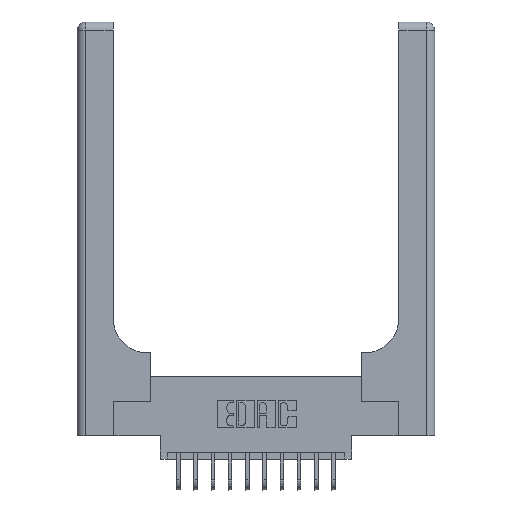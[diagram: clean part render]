
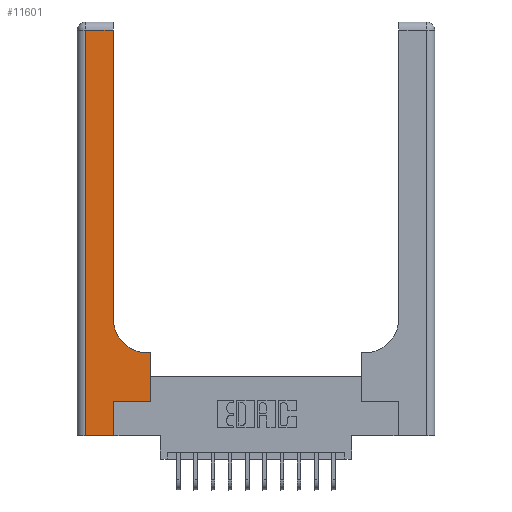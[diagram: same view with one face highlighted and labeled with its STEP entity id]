
A CAD part, top view. The second image highlights one B-rep face of the part: STEP entity #11601.
In plain terms, the highlighted planar face has unit normal (0, 0, 1).
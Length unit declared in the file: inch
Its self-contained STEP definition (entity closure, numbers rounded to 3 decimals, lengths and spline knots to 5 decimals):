
#465 = DIRECTION ( 'NONE',  ( 0., 1., 0. ) ) ;
#601 = PLANE ( 'NONE',  #8319 ) ;
#725 = ORIENTED_EDGE ( 'NONE', *, *, #13886, .T. ) ;
#1067 = EDGE_LOOP ( 'NONE', ( #1439, #725, #13092, #6729, #8405, #2641, #15620, #2859, #9228 ) ) ;
#1168 = VECTOR ( 'NONE', #14982, 39.37008 ) ;
#1403 = VERTEX_POINT ( 'NONE', #11383 ) ;
#1439 = ORIENTED_EDGE ( 'NONE', *, *, #6930, .T. ) ;
#1854 = LINE ( 'NONE', #16345, #11852 ) ;
#1896 = CIRCLE ( 'NONE', #6015, 0.25 ) ;
#2641 = ORIENTED_EDGE ( 'NONE', *, *, #15025, .T. ) ;
#2706 = EDGE_CURVE ( 'NONE', #8945, #14897, #8207, .T. ) ;
#2821 = VERTEX_POINT ( 'NONE', #8493 ) ;
#2859 = ORIENTED_EDGE ( 'NONE', *, *, #18335, .T. ) ;
#2929 = CARTESIAN_POINT ( 'NONE',  ( 0.265, 0.25, 0.37 ) ) ;
#3144 = CARTESIAN_POINT ( 'NONE',  ( 0.26, 2.94, 0.37 ) ) ;
#3478 = CARTESIAN_POINT ( 'NONE',  ( 0., 3., 0.37 ) ) ;
#3598 = LINE ( 'NONE', #9259, #17784 ) ;
#3616 = DIRECTION ( 'NONE',  ( -1., 0., 0. ) ) ;
#3649 = CARTESIAN_POINT ( 'NONE',  ( 0.26, 3., 0.37 ) ) ;
#3836 = CARTESIAN_POINT ( 'NONE',  ( 0.51, 0.85, 0.37 ) ) ;
#3885 = DIRECTION ( 'NONE',  ( 0., -1., 0. ) ) ;
#5027 = CARTESIAN_POINT ( 'NONE',  ( 0., 0., 0.37 ) ) ;
#5035 = FACE_OUTER_BOUND ( 'NONE', #1067, .T. ) ;
#5143 = DIRECTION ( 'NONE',  ( 0., 0., -1. ) ) ;
#5340 = VERTEX_POINT ( 'NONE', #8844 ) ;
#5432 = VERTEX_POINT ( 'NONE', #10912 ) ;
#6015 = AXIS2_PLACEMENT_3D ( 'NONE', #3836, #5143, #6525 ) ;
#6072 = VECTOR ( 'NONE', #16214, 39.37008 ) ;
#6525 = DIRECTION ( 'NONE',  ( 1., 0., 0. ) ) ;
#6729 = ORIENTED_EDGE ( 'NONE', *, *, #18105, .T. ) ;
#6781 = LINE ( 'NONE', #5027, #1168 ) ;
#6930 = EDGE_CURVE ( 'NONE', #17039, #15753, #14693, .T. ) ;
#7215 = VECTOR ( 'NONE', #3885, 39.37008 ) ;
#7459 = LINE ( 'NONE', #9058, #6072 ) ;
#7464 = VECTOR ( 'NONE', #465, 39.37008 ) ;
#8068 = LINE ( 'NONE', #16622, #7215 ) ;
#8126 = VECTOR ( 'NONE', #10970, 39.37008 ) ;
#8207 = LINE ( 'NONE', #15881, #7464 ) ;
#8314 = VERTEX_POINT ( 'NONE', #14802 ) ;
#8319 = AXIS2_PLACEMENT_3D ( 'NONE', #3478, #12017, #9327 ) ;
#8405 = ORIENTED_EDGE ( 'NONE', *, *, #2706, .T. ) ;
#8430 = EDGE_CURVE ( 'NONE', #8314, #17039, #1896, .T. ) ;
#8493 = CARTESIAN_POINT ( 'NONE',  ( 0.528, 0.25, 0.37 ) ) ;
#8844 = CARTESIAN_POINT ( 'NONE',  ( 0.06, 2.94, 0.37 ) ) ;
#8929 = EDGE_CURVE ( 'NONE', #2821, #5432, #18118, .T. ) ;
#8934 = EDGE_CURVE ( 'NONE', #5340, #1403, #8068, .T. ) ;
#8945 = VERTEX_POINT ( 'NONE', #17265 ) ;
#9058 = CARTESIAN_POINT ( 'NONE',  ( 0.265, 0.25, 0.37 ) ) ;
#9228 = ORIENTED_EDGE ( 'NONE', *, *, #8430, .T. ) ;
#9259 = CARTESIAN_POINT ( 'NONE',  ( 0., 2.94, 0.37 ) ) ;
#9327 = DIRECTION ( 'NONE',  ( -1., 0., 0. ) ) ;
#9477 = CARTESIAN_POINT ( 'NONE',  ( 0.528, 0.25, 0.37 ) ) ;
#10912 = CARTESIAN_POINT ( 'NONE',  ( 0.528, 0.6, 0.37 ) ) ;
#10970 = DIRECTION ( 'NONE',  ( 0., 1., 0. ) ) ;
#11383 = CARTESIAN_POINT ( 'NONE',  ( 0.06, 0., 0.37 ) ) ;
#11601 = ADVANCED_FACE ( 'NONE', ( #5035 ), #601, .F. ) ;
#11852 = VECTOR ( 'NONE', #3616, 39.37008 ) ;
#12017 = DIRECTION ( 'NONE',  ( 0., 0., -1. ) ) ;
#13088 = VECTOR ( 'NONE', #13380, 39.37008 ) ;
#13092 = ORIENTED_EDGE ( 'NONE', *, *, #8934, .T. ) ;
#13380 = DIRECTION ( 'NONE',  ( 0., 1., 0. ) ) ;
#13886 = EDGE_CURVE ( 'NONE', #15753, #5340, #3598, .T. ) ;
#14693 = LINE ( 'NONE', #3649, #13088 ) ;
#14802 = CARTESIAN_POINT ( 'NONE',  ( 0.51, 0.6, 0.37 ) ) ;
#14897 = VERTEX_POINT ( 'NONE', #2929 ) ;
#14923 = DIRECTION ( 'NONE',  ( -1., 0., 0. ) ) ;
#14982 = DIRECTION ( 'NONE',  ( 1., 0., 0. ) ) ;
#15025 = EDGE_CURVE ( 'NONE', #14897, #2821, #7459, .T. ) ;
#15620 = ORIENTED_EDGE ( 'NONE', *, *, #8929, .T. ) ;
#15753 = VERTEX_POINT ( 'NONE', #3144 ) ;
#15881 = CARTESIAN_POINT ( 'NONE',  ( 0.265, 0., 0.37 ) ) ;
#16214 = DIRECTION ( 'NONE',  ( 1., 0., 0. ) ) ;
#16345 = CARTESIAN_POINT ( 'NONE',  ( 0.26, 0.6, 0.37 ) ) ;
#16622 = CARTESIAN_POINT ( 'NONE',  ( 0.06, 3., 0.37 ) ) ;
#17015 = CARTESIAN_POINT ( 'NONE',  ( 0.26, 0.85, 0.37 ) ) ;
#17039 = VERTEX_POINT ( 'NONE', #17015 ) ;
#17265 = CARTESIAN_POINT ( 'NONE',  ( 0.265, 0., 0.37 ) ) ;
#17784 = VECTOR ( 'NONE', #14923, 39.37008 ) ;
#18105 = EDGE_CURVE ( 'NONE', #1403, #8945, #6781, .T. ) ;
#18118 = LINE ( 'NONE', #9477, #8126 ) ;
#18335 = EDGE_CURVE ( 'NONE', #5432, #8314, #1854, .T. ) ;
